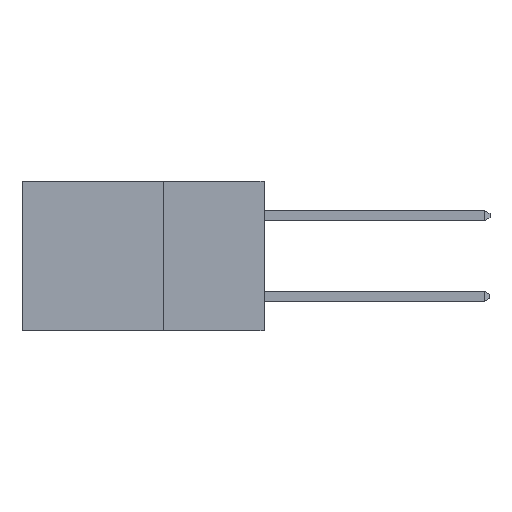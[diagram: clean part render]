
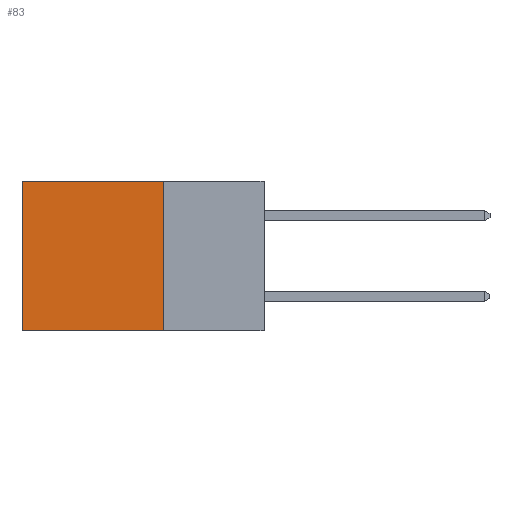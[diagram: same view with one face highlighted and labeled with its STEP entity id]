
A CAD part, left-side view. The second image highlights one B-rep face of the part: STEP entity #83.
In plain terms, the highlighted planar face has unit normal (-1, 0, 0).
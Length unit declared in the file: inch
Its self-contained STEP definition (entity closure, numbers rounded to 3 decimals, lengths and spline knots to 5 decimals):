
#83 = ADVANCED_FACE ( 'NONE', ( #6188 ), #7515, .F. ) ;
#84 = CARTESIAN_POINT ( 'NONE',  ( 0.2615, 0.25, -0.37 ) ) ;
#109 = DIRECTION ( 'NONE',  ( 0., 0., -1. ) ) ;
#157 = ORIENTED_EDGE ( 'NONE', *, *, #3354, .F. ) ;
#563 = EDGE_CURVE ( 'NONE', #8633, #4032, #4148, .T. ) ;
#1194 = CARTESIAN_POINT ( 'NONE',  ( 0.2615, 0.25, 0. ) ) ;
#1509 = LINE ( 'NONE', #7791, #6267 ) ;
#1517 = EDGE_LOOP ( 'NONE', ( #3415, #3302, #157, #3051 ) ) ;
#1730 = VECTOR ( 'NONE', #6945, 39.37008 ) ;
#2439 = AXIS2_PLACEMENT_3D ( 'NONE', #4868, #6145, #8285 ) ;
#2529 = CARTESIAN_POINT ( 'NONE',  ( 0.2615, 0.25, 0. ) ) ;
#3051 = ORIENTED_EDGE ( 'NONE', *, *, #563, .T. ) ;
#3254 = CARTESIAN_POINT ( 'NONE',  ( 0.2615, 0.25, -0.37 ) ) ;
#3302 = ORIENTED_EDGE ( 'NONE', *, *, #4424, .F. ) ;
#3354 = EDGE_CURVE ( 'NONE', #8633, #4241, #1509, .T. ) ;
#3415 = ORIENTED_EDGE ( 'NONE', *, *, #4943, .T. ) ;
#3942 = VECTOR ( 'NONE', #4455, 39.37008 ) ;
#4032 = VERTEX_POINT ( 'NONE', #7588 ) ;
#4148 = LINE ( 'NONE', #2529, #1730 ) ;
#4241 = VERTEX_POINT ( 'NONE', #84 ) ;
#4424 = EDGE_CURVE ( 'NONE', #4241, #6682, #8670, .T. ) ;
#4455 = DIRECTION ( 'NONE',  ( 0., 1., 0. ) ) ;
#4868 = CARTESIAN_POINT ( 'NONE',  ( 0.2615, 0.25, -0.37 ) ) ;
#4943 = EDGE_CURVE ( 'NONE', #4032, #6682, #6600, .T. ) ;
#5277 = VECTOR ( 'NONE', #8692, 39.37008 ) ;
#5776 = CARTESIAN_POINT ( 'NONE',  ( 0.2615, 0.6, -0.37 ) ) ;
#6145 = DIRECTION ( 'NONE',  ( 1., 0., 0. ) ) ;
#6188 = FACE_OUTER_BOUND ( 'NONE', #1517, .T. ) ;
#6267 = VECTOR ( 'NONE', #109, 39.37008 ) ;
#6600 = LINE ( 'NONE', #5776, #5277 ) ;
#6682 = VERTEX_POINT ( 'NONE', #8002 ) ;
#6945 = DIRECTION ( 'NONE',  ( 0., 1., 0. ) ) ;
#7515 = PLANE ( 'NONE',  #2439 ) ;
#7588 = CARTESIAN_POINT ( 'NONE',  ( 0.2615, 0.6, 0. ) ) ;
#7791 = CARTESIAN_POINT ( 'NONE',  ( 0.2615, 0.25, -0.37 ) ) ;
#8002 = CARTESIAN_POINT ( 'NONE',  ( 0.2615, 0.6, -0.37 ) ) ;
#8285 = DIRECTION ( 'NONE',  ( 0., 0., -1. ) ) ;
#8633 = VERTEX_POINT ( 'NONE', #1194 ) ;
#8670 = LINE ( 'NONE', #3254, #3942 ) ;
#8692 = DIRECTION ( 'NONE',  ( 0., 0., -1. ) ) ;
